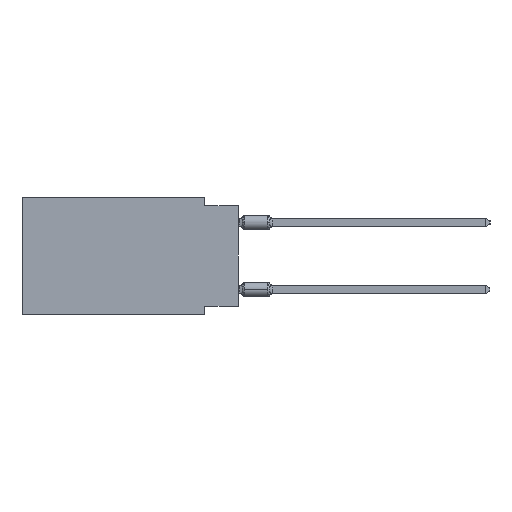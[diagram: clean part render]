
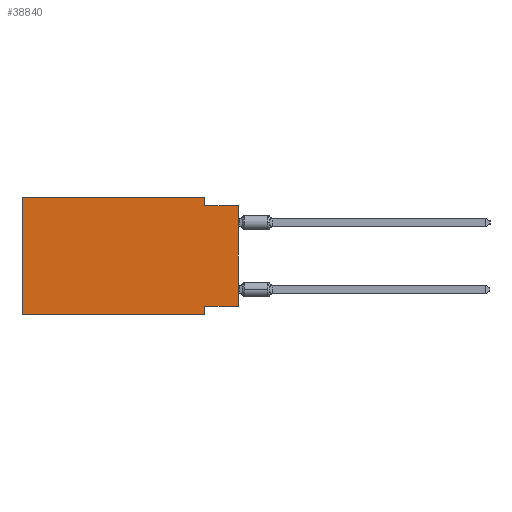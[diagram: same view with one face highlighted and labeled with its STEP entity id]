
A CAD part, left-side view. The second image highlights one B-rep face of the part: STEP entity #38840.
In plain terms, the highlighted planar face has unit normal (-1, 0, 0).
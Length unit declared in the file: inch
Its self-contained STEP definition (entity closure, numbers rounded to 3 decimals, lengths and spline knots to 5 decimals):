
#1379 = CARTESIAN_POINT ( 'NONE',  ( 0., 0.1, -0.025 ) ) ;
#3141 = VECTOR ( 'NONE', #7955, 39.37008 ) ;
#4506 = LINE ( 'NONE', #23800, #57226 ) ;
#5687 = CARTESIAN_POINT ( 'NONE',  ( 0., 0.645, 0. ) ) ;
#6251 = CARTESIAN_POINT ( 'NONE',  ( 0., 0., 0. ) ) ;
#6645 = EDGE_CURVE ( 'NONE', #51876, #56501, #47384, .T. ) ;
#6864 = ORIENTED_EDGE ( 'NONE', *, *, #34354, .F. ) ;
#7824 = CARTESIAN_POINT ( 'NONE',  ( 0., 0., -0.325 ) ) ;
#7955 = DIRECTION ( 'NONE',  ( 0., 0., -1. ) ) ;
#9505 = CARTESIAN_POINT ( 'NONE',  ( 0., 0.645, -0.35 ) ) ;
#10669 = VECTOR ( 'NONE', #12290, 39.37008 ) ;
#11055 = EDGE_CURVE ( 'NONE', #51876, #11674, #30919, .T. ) ;
#11674 = VERTEX_POINT ( 'NONE', #23760 ) ;
#12290 = DIRECTION ( 'NONE',  ( 0., -1., 0. ) ) ;
#13923 = EDGE_CURVE ( 'NONE', #56272, #19737, #38315, .T. ) ;
#14312 = DIRECTION ( 'NONE',  ( 0., 0., -1. ) ) ;
#14629 = DIRECTION ( 'NONE',  ( 1., 0., 0. ) ) ;
#16519 = CARTESIAN_POINT ( 'NONE',  ( 0., 0.1, -0.35 ) ) ;
#17500 = CARTESIAN_POINT ( 'NONE',  ( 0., 0.1, 0. ) ) ;
#17530 = EDGE_CURVE ( 'NONE', #35277, #61603, #28113, .T. ) ;
#18562 = DIRECTION ( 'NONE',  ( 0., 1., 0. ) ) ;
#19363 = FACE_OUTER_BOUND ( 'NONE', #45336, .T. ) ;
#19737 = VERTEX_POINT ( 'NONE', #33399 ) ;
#22081 = CARTESIAN_POINT ( 'NONE',  ( 0., 0., -0.025 ) ) ;
#23760 = CARTESIAN_POINT ( 'NONE',  ( 0., 0., -0.025 ) ) ;
#23800 = CARTESIAN_POINT ( 'NONE',  ( 0., 0.645, 0. ) ) ;
#24123 = PLANE ( 'NONE',  #37369 ) ;
#24657 = ORIENTED_EDGE ( 'NONE', *, *, #13923, .T. ) ;
#26082 = VECTOR ( 'NONE', #34504, 39.37008 ) ;
#27650 = LINE ( 'NONE', #47602, #29801 ) ;
#27683 = EDGE_CURVE ( 'NONE', #61603, #11674, #36331, .T. ) ;
#28113 = LINE ( 'NONE', #36994, #48649 ) ;
#29801 = VECTOR ( 'NONE', #32722, 39.37008 ) ;
#30919 = LINE ( 'NONE', #6251, #56293 ) ;
#32244 = ORIENTED_EDGE ( 'NONE', *, *, #11055, .T. ) ;
#32722 = DIRECTION ( 'NONE',  ( 0., -1., 0. ) ) ;
#33399 = CARTESIAN_POINT ( 'NONE',  ( 0., 0.1, -0.35 ) ) ;
#33573 = ORIENTED_EDGE ( 'NONE', *, *, #27683, .F. ) ;
#34354 = EDGE_CURVE ( 'NONE', #56501, #19737, #53584, .T. ) ;
#34504 = DIRECTION ( 'NONE',  ( 0., -1., 0. ) ) ;
#35277 = VERTEX_POINT ( 'NONE', #17500 ) ;
#36331 = LINE ( 'NONE', #22081, #10669 ) ;
#36994 = CARTESIAN_POINT ( 'NONE',  ( 0., 0.1, 0. ) ) ;
#37369 = AXIS2_PLACEMENT_3D ( 'NONE', #58004, #14629, #14312 ) ;
#38315 = LINE ( 'NONE', #9505, #26082 ) ;
#38840 = ADVANCED_FACE ( 'NONE', ( #19363 ), #24123, .F. ) ;
#40576 = ORIENTED_EDGE ( 'NONE', *, *, #17530, .F. ) ;
#43131 = DIRECTION ( 'NONE',  ( 0., 0., 1. ) ) ;
#45336 = EDGE_LOOP ( 'NONE', ( #32244, #33573, #40576, #50837, #54120, #24657, #6864, #48868 ) ) ;
#47384 = LINE ( 'NONE', #7824, #61920 ) ;
#47602 = CARTESIAN_POINT ( 'NONE',  ( 0., 0.645, 0. ) ) ;
#47998 = EDGE_CURVE ( 'NONE', #56272, #48509, #4506, .T. ) ;
#48509 = VERTEX_POINT ( 'NONE', #5687 ) ;
#48649 = VECTOR ( 'NONE', #57263, 39.37008 ) ;
#48764 = CARTESIAN_POINT ( 'NONE',  ( 0., 0., -0.325 ) ) ;
#48868 = ORIENTED_EDGE ( 'NONE', *, *, #6645, .F. ) ;
#50837 = ORIENTED_EDGE ( 'NONE', *, *, #56969, .F. ) ;
#51876 = VERTEX_POINT ( 'NONE', #48764 ) ;
#52672 = CARTESIAN_POINT ( 'NONE',  ( 0., 0.645, -0.35 ) ) ;
#53584 = LINE ( 'NONE', #16519, #3141 ) ;
#54120 = ORIENTED_EDGE ( 'NONE', *, *, #47998, .F. ) ;
#56103 = CARTESIAN_POINT ( 'NONE',  ( 0., 0.1, -0.325 ) ) ;
#56272 = VERTEX_POINT ( 'NONE', #52672 ) ;
#56293 = VECTOR ( 'NONE', #59451, 39.37008 ) ;
#56501 = VERTEX_POINT ( 'NONE', #56103 ) ;
#56969 = EDGE_CURVE ( 'NONE', #48509, #35277, #27650, .T. ) ;
#57226 = VECTOR ( 'NONE', #43131, 39.37008 ) ;
#57263 = DIRECTION ( 'NONE',  ( 0., 0., -1. ) ) ;
#58004 = CARTESIAN_POINT ( 'NONE',  ( 0., 0.645, 0. ) ) ;
#59451 = DIRECTION ( 'NONE',  ( 0., 0., 1. ) ) ;
#61603 = VERTEX_POINT ( 'NONE', #1379 ) ;
#61920 = VECTOR ( 'NONE', #18562, 39.37008 ) ;
